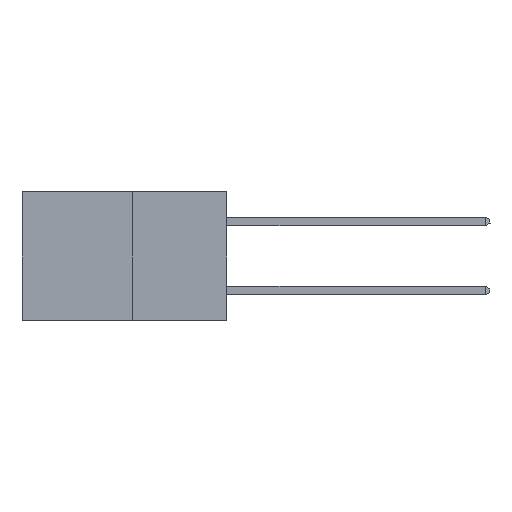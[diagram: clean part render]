
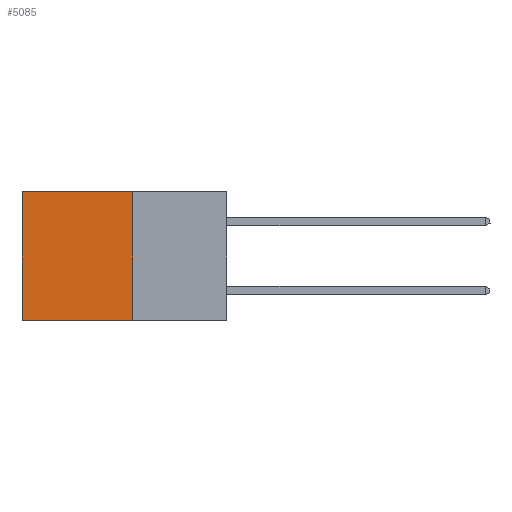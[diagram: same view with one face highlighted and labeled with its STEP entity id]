
A CAD part, left-side view. The second image highlights one B-rep face of the part: STEP entity #5085.
In plain terms, the highlighted planar face has unit normal (-1, 0, 0).
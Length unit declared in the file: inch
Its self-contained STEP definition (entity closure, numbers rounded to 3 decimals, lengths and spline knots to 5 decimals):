
#192 = EDGE_LOOP ( 'NONE', ( #1106, #3498, #9822, #1716 ) ) ;
#767 = LINE ( 'NONE', #1778, #1030 ) ;
#894 = DIRECTION ( 'NONE',  ( 0., 0., -1. ) ) ;
#1030 = VECTOR ( 'NONE', #2388, 39.37008 ) ;
#1106 = ORIENTED_EDGE ( 'NONE', *, *, #4479, .T. ) ;
#1259 = CARTESIAN_POINT ( 'NONE',  ( 0.277, 0.27, 0. ) ) ;
#1562 = LINE ( 'NONE', #9561, #8033 ) ;
#1647 = VECTOR ( 'NONE', #3884, 39.37008 ) ;
#1716 = ORIENTED_EDGE ( 'NONE', *, *, #5063, .T. ) ;
#1778 = CARTESIAN_POINT ( 'NONE',  ( 0.277, 0.27, 0. ) ) ;
#2388 = DIRECTION ( 'NONE',  ( 0., 1., 0. ) ) ;
#2940 = EDGE_CURVE ( 'NONE', #9603, #8117, #7573, .T. ) ;
#3242 = CARTESIAN_POINT ( 'NONE',  ( 0.277, 0.27, -0.37 ) ) ;
#3337 = PLANE ( 'NONE',  #9857 ) ;
#3498 = ORIENTED_EDGE ( 'NONE', *, *, #7922, .F. ) ;
#3884 = DIRECTION ( 'NONE',  ( 0., 1., 0. ) ) ;
#4298 = VERTEX_POINT ( 'NONE', #5624 ) ;
#4479 = EDGE_CURVE ( 'NONE', #4298, #7542, #1562, .T. ) ;
#4896 = FACE_OUTER_BOUND ( 'NONE', #192, .T. ) ;
#5063 = EDGE_CURVE ( 'NONE', #9603, #4298, #767, .T. ) ;
#5085 = ADVANCED_FACE ( 'NONE', ( #4896 ), #3337, .F. ) ;
#5455 = DIRECTION ( 'NONE',  ( 1., 0., 0. ) ) ;
#5471 = VECTOR ( 'NONE', #894, 39.37008 ) ;
#5624 = CARTESIAN_POINT ( 'NONE',  ( 0.277, 0.59, 0. ) ) ;
#6242 = LINE ( 'NONE', #3242, #1647 ) ;
#6525 = DIRECTION ( 'NONE',  ( 0., 0., -1. ) ) ;
#7542 = VERTEX_POINT ( 'NONE', #8732 ) ;
#7573 = LINE ( 'NONE', #9984, #5471 ) ;
#7695 = CARTESIAN_POINT ( 'NONE',  ( 0.277, 0.27, -0.37 ) ) ;
#7922 = EDGE_CURVE ( 'NONE', #8117, #7542, #6242, .T. ) ;
#8033 = VECTOR ( 'NONE', #9308, 39.37008 ) ;
#8117 = VERTEX_POINT ( 'NONE', #7695 ) ;
#8732 = CARTESIAN_POINT ( 'NONE',  ( 0.277, 0.59, -0.37 ) ) ;
#9146 = CARTESIAN_POINT ( 'NONE',  ( 0.277, 0.27, -0.37 ) ) ;
#9308 = DIRECTION ( 'NONE',  ( 0., 0., -1. ) ) ;
#9561 = CARTESIAN_POINT ( 'NONE',  ( 0.277, 0.59, -0.37 ) ) ;
#9603 = VERTEX_POINT ( 'NONE', #1259 ) ;
#9822 = ORIENTED_EDGE ( 'NONE', *, *, #2940, .F. ) ;
#9857 = AXIS2_PLACEMENT_3D ( 'NONE', #9146, #5455, #6525 ) ;
#9984 = CARTESIAN_POINT ( 'NONE',  ( 0.277, 0.27, -0.37 ) ) ;
